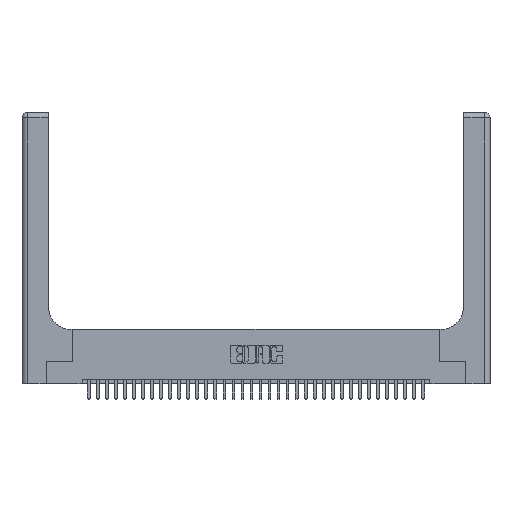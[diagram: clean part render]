
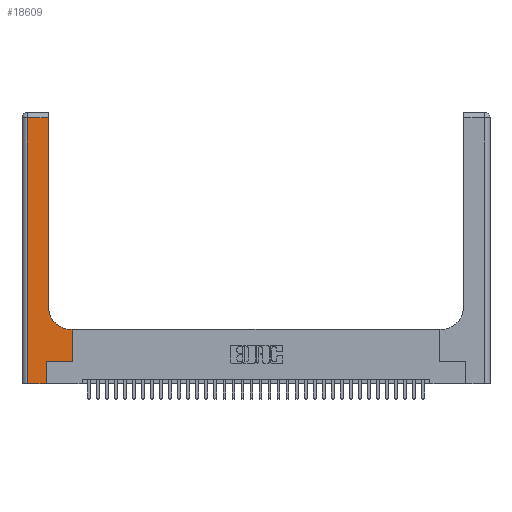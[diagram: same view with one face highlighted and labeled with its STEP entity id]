
A CAD part, top view. The second image highlights one B-rep face of the part: STEP entity #18609.
In plain terms, the highlighted planar face has unit normal (0, 0, 1).
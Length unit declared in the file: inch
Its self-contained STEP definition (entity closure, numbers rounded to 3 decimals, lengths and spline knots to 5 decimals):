
#57 = EDGE_CURVE ( 'NONE', #4947, #9480, #16465, .T. ) ;
#792 = VECTOR ( 'NONE', #13962, 39.37008 ) ;
#1089 = CARTESIAN_POINT ( 'NONE',  ( 0.269, 0.25, 0.37 ) ) ;
#1469 = ORIENTED_EDGE ( 'NONE', *, *, #5528, .T. ) ;
#1684 = CARTESIAN_POINT ( 'NONE',  ( 0.2915, 3., 0.37 ) ) ;
#1834 = EDGE_CURVE ( 'NONE', #21223, #4947, #9931, .T. ) ;
#2633 = CARTESIAN_POINT ( 'NONE',  ( 0.5585, 0.25, 0.37 ) ) ;
#3274 = AXIS2_PLACEMENT_3D ( 'NONE', #9891, #29007, #12694 ) ;
#3747 = ORIENTED_EDGE ( 'NONE', *, *, #31879, .T. ) ;
#3794 = ORIENTED_EDGE ( 'NONE', *, *, #25005, .T. ) ;
#4038 = CARTESIAN_POINT ( 'NONE',  ( 0.06, 3., 0.37 ) ) ;
#4066 = VECTOR ( 'NONE', #15278, 39.37008 ) ;
#4947 = VERTEX_POINT ( 'NONE', #18907 ) ;
#5528 = EDGE_CURVE ( 'NONE', #31018, #21223, #14696, .T. ) ;
#5550 = CARTESIAN_POINT ( 'NONE',  ( 0.2915, 0.6, 0.37 ) ) ;
#5735 = VERTEX_POINT ( 'NONE', #29993 ) ;
#5795 = VERTEX_POINT ( 'NONE', #22096 ) ;
#6105 = ORIENTED_EDGE ( 'NONE', *, *, #1834, .T. ) ;
#7260 = CARTESIAN_POINT ( 'NONE',  ( 0., 0., 0.37 ) ) ;
#7862 = AXIS2_PLACEMENT_3D ( 'NONE', #9672, #28798, #12473 ) ;
#8201 = VECTOR ( 'NONE', #23797, 39.37008 ) ;
#8424 = LINE ( 'NONE', #2633, #792 ) ;
#9265 = CARTESIAN_POINT ( 'NONE',  ( 0.5585, 0.6, 0.37 ) ) ;
#9480 = VERTEX_POINT ( 'NONE', #28193 ) ;
#9525 = VERTEX_POINT ( 'NONE', #9265 ) ;
#9672 = CARTESIAN_POINT ( 'NONE',  ( 0.5415, 0.85, 0.37 ) ) ;
#9891 = CARTESIAN_POINT ( 'NONE',  ( 0., 3., 0.37 ) ) ;
#9931 = LINE ( 'NONE', #20749, #23704 ) ;
#10099 = CARTESIAN_POINT ( 'NONE',  ( 0.269, 0., 0.37 ) ) ;
#10657 = ORIENTED_EDGE ( 'NONE', *, *, #23817, .T. ) ;
#12473 = DIRECTION ( 'NONE',  ( 1., 0., 0. ) ) ;
#12694 = DIRECTION ( 'NONE',  ( -1., 0., 0. ) ) ;
#13755 = DIRECTION ( 'NONE',  ( -1., 0., 0. ) ) ;
#13962 = DIRECTION ( 'NONE',  ( 0., 1., 0. ) ) ;
#14268 = ORIENTED_EDGE ( 'NONE', *, *, #30841, .T. ) ;
#14431 = CARTESIAN_POINT ( 'NONE',  ( 0.06, 2.94, 0.37 ) ) ;
#14696 = LINE ( 'NONE', #7260, #8201 ) ;
#15278 = DIRECTION ( 'NONE',  ( 0., -1., 0. ) ) ;
#16465 = LINE ( 'NONE', #1089, #24634 ) ;
#17699 = ORIENTED_EDGE ( 'NONE', *, *, #34807, .T. ) ;
#18099 = DIRECTION ( 'NONE',  ( 0., 1., 0. ) ) ;
#18241 = LINE ( 'NONE', #24785, #32647 ) ;
#18574 = DIRECTION ( 'NONE',  ( 0., 1., 0. ) ) ;
#18609 = ADVANCED_FACE ( 'NONE', ( #31769 ), #31581, .F. ) ;
#18907 = CARTESIAN_POINT ( 'NONE',  ( 0.269, 0.25, 0.37 ) ) ;
#20535 = EDGE_CURVE ( 'NONE', #5795, #5735, #30811, .T. ) ;
#20749 = CARTESIAN_POINT ( 'NONE',  ( 0.269, 0., 0.37 ) ) ;
#21223 = VERTEX_POINT ( 'NONE', #10099 ) ;
#22096 = CARTESIAN_POINT ( 'NONE',  ( 0.2915, 0.85, 0.37 ) ) ;
#22207 = VERTEX_POINT ( 'NONE', #25103 ) ;
#22876 = LINE ( 'NONE', #5550, #23746 ) ;
#23704 = VECTOR ( 'NONE', #18099, 39.37008 ) ;
#23746 = VECTOR ( 'NONE', #27575, 39.37008 ) ;
#23797 = DIRECTION ( 'NONE',  ( 1., 0., 0. ) ) ;
#23817 = EDGE_CURVE ( 'NONE', #25682, #31018, #29770, .T. ) ;
#24360 = CARTESIAN_POINT ( 'NONE',  ( 0.06, 0., 0.37 ) ) ;
#24634 = VECTOR ( 'NONE', #27077, 39.37008 ) ;
#24785 = CARTESIAN_POINT ( 'NONE',  ( 0., 2.94, 0.37 ) ) ;
#25005 = EDGE_CURVE ( 'NONE', #5735, #25682, #18241, .T. ) ;
#25103 = CARTESIAN_POINT ( 'NONE',  ( 0.5415, 0.6, 0.37 ) ) ;
#25682 = VERTEX_POINT ( 'NONE', #14431 ) ;
#25899 = ORIENTED_EDGE ( 'NONE', *, *, #20535, .T. ) ;
#27077 = DIRECTION ( 'NONE',  ( 1., 0., 0. ) ) ;
#27249 = EDGE_LOOP ( 'NONE', ( #25899, #3794, #10657, #1469, #6105, #30910, #17699, #3747, #14268 ) ) ;
#27575 = DIRECTION ( 'NONE',  ( -1., 0., 0. ) ) ;
#28193 = CARTESIAN_POINT ( 'NONE',  ( 0.5585, 0.25, 0.37 ) ) ;
#28798 = DIRECTION ( 'NONE',  ( 0., 0., -1. ) ) ;
#29007 = DIRECTION ( 'NONE',  ( 0., 0., -1. ) ) ;
#29770 = LINE ( 'NONE', #4038, #4066 ) ;
#29989 = VECTOR ( 'NONE', #18574, 39.37008 ) ;
#29993 = CARTESIAN_POINT ( 'NONE',  ( 0.2915, 2.94, 0.37 ) ) ;
#30811 = LINE ( 'NONE', #1684, #29989 ) ;
#30841 = EDGE_CURVE ( 'NONE', #22207, #5795, #33477, .T. ) ;
#30910 = ORIENTED_EDGE ( 'NONE', *, *, #57, .T. ) ;
#31018 = VERTEX_POINT ( 'NONE', #24360 ) ;
#31581 = PLANE ( 'NONE',  #3274 ) ;
#31769 = FACE_OUTER_BOUND ( 'NONE', #27249, .T. ) ;
#31879 = EDGE_CURVE ( 'NONE', #9525, #22207, #22876, .T. ) ;
#32647 = VECTOR ( 'NONE', #13755, 39.37008 ) ;
#33477 = CIRCLE ( 'NONE', #7862, 0.25 ) ;
#34807 = EDGE_CURVE ( 'NONE', #9480, #9525, #8424, .T. ) ;
